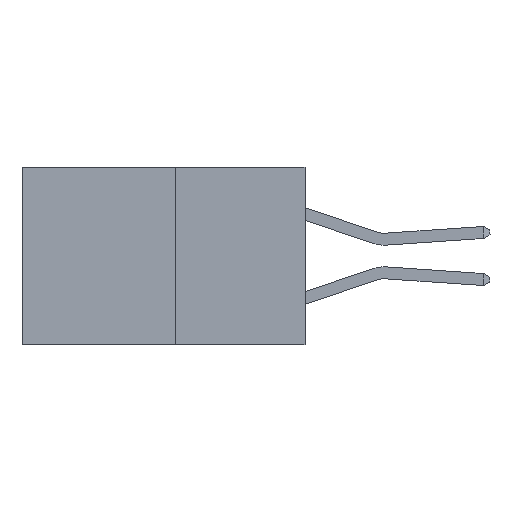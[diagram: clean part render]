
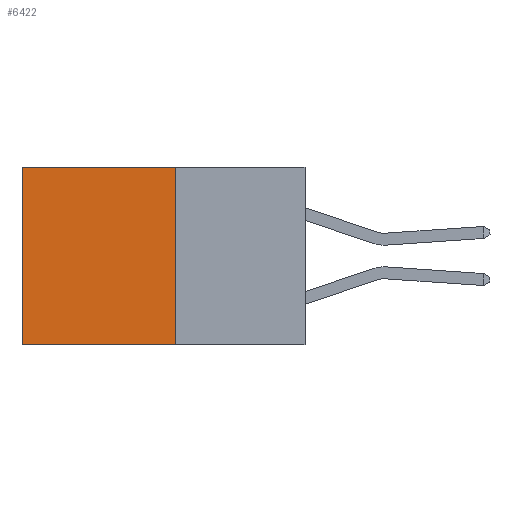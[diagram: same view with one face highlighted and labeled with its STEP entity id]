
A CAD part, left-side view. The second image highlights one B-rep face of the part: STEP entity #6422.
In plain terms, the highlighted planar face has unit normal (-1, 0, 0).
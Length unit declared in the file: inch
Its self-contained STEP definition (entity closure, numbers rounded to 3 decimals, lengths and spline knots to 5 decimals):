
#110 = EDGE_CURVE ( 'NONE', #8761, #2456, #9699, .T. ) ;
#167 = VERTEX_POINT ( 'NONE', #9620 ) ;
#424 = EDGE_CURVE ( 'NONE', #7285, #167, #4081, .T. ) ;
#629 = VECTOR ( 'NONE', #5308, 39.37008 ) ;
#1488 = CARTESIAN_POINT ( 'NONE',  ( 0.277, 0.27, -0.37 ) ) ;
#1834 = AXIS2_PLACEMENT_3D ( 'NONE', #3658, #3971, #4646 ) ;
#1868 = VECTOR ( 'NONE', #9187, 39.37008 ) ;
#1901 = CARTESIAN_POINT ( 'NONE',  ( 0.277, 0.27, -0.37 ) ) ;
#1917 = VECTOR ( 'NONE', #7912, 39.37008 ) ;
#2236 = EDGE_CURVE ( 'NONE', #7285, #8761, #2973, .T. ) ;
#2411 = EDGE_CURVE ( 'NONE', #167, #2456, #3799, .T. ) ;
#2456 = VERTEX_POINT ( 'NONE', #9813 ) ;
#2615 = ORIENTED_EDGE ( 'NONE', *, *, #424, .F. ) ;
#2846 = ORIENTED_EDGE ( 'NONE', *, *, #2411, .F. ) ;
#2973 = LINE ( 'NONE', #5150, #629 ) ;
#3463 = CARTESIAN_POINT ( 'NONE',  ( 0.277, 0.59, -0.37 ) ) ;
#3658 = CARTESIAN_POINT ( 'NONE',  ( 0.277, 0.27, -0.37 ) ) ;
#3799 = LINE ( 'NONE', #1488, #1868 ) ;
#3971 = DIRECTION ( 'NONE',  ( 1., 0., 0. ) ) ;
#4081 = LINE ( 'NONE', #1901, #1917 ) ;
#4614 = ORIENTED_EDGE ( 'NONE', *, *, #2236, .T. ) ;
#4646 = DIRECTION ( 'NONE',  ( 0., 0., -1. ) ) ;
#4871 = DIRECTION ( 'NONE',  ( 0., 0., -1. ) ) ;
#4913 = CARTESIAN_POINT ( 'NONE',  ( 0.277, 0.59, 0. ) ) ;
#5150 = CARTESIAN_POINT ( 'NONE',  ( 0.277, 0.27, 0. ) ) ;
#5308 = DIRECTION ( 'NONE',  ( 0., 1., 0. ) ) ;
#5475 = VECTOR ( 'NONE', #4871, 39.37008 ) ;
#5518 = EDGE_LOOP ( 'NONE', ( #6590, #2846, #2615, #4614 ) ) ;
#6422 = ADVANCED_FACE ( 'NONE', ( #8223 ), #8514, .F. ) ;
#6590 = ORIENTED_EDGE ( 'NONE', *, *, #110, .T. ) ;
#7285 = VERTEX_POINT ( 'NONE', #7931 ) ;
#7912 = DIRECTION ( 'NONE',  ( 0., 0., -1. ) ) ;
#7931 = CARTESIAN_POINT ( 'NONE',  ( 0.277, 0.27, 0. ) ) ;
#8223 = FACE_OUTER_BOUND ( 'NONE', #5518, .T. ) ;
#8514 = PLANE ( 'NONE',  #1834 ) ;
#8761 = VERTEX_POINT ( 'NONE', #4913 ) ;
#9187 = DIRECTION ( 'NONE',  ( 0., 1., 0. ) ) ;
#9620 = CARTESIAN_POINT ( 'NONE',  ( 0.277, 0.27, -0.37 ) ) ;
#9699 = LINE ( 'NONE', #3463, #5475 ) ;
#9813 = CARTESIAN_POINT ( 'NONE',  ( 0.277, 0.59, -0.37 ) ) ;
